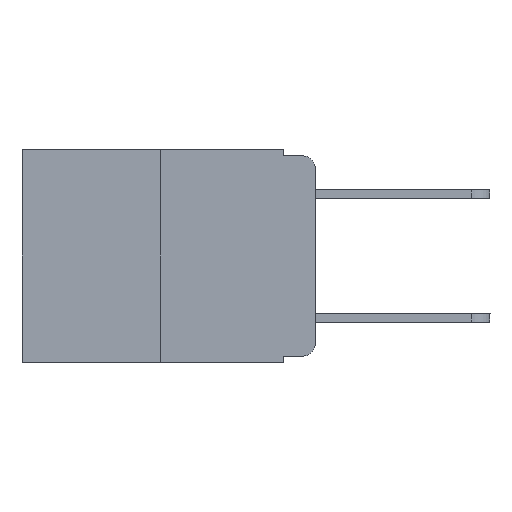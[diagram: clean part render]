
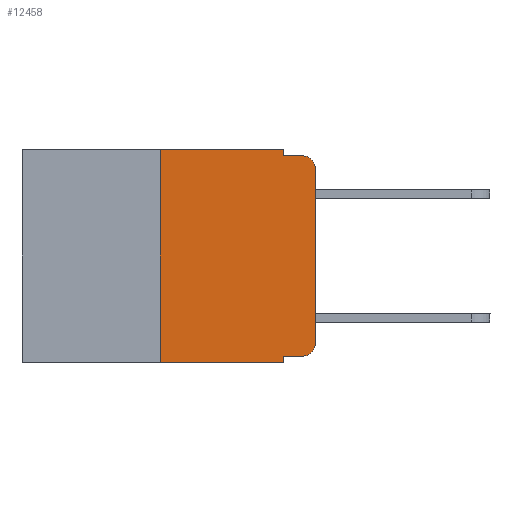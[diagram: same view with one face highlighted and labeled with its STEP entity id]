
A CAD part, left-side view. The second image highlights one B-rep face of the part: STEP entity #12458.
In plain terms, the highlighted planar face has unit normal (-1, 0, 0).
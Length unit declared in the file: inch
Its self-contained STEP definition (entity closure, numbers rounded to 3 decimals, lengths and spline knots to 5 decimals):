
#30 = ORIENTED_EDGE ( 'NONE', *, *, #13722, .T. ) ;
#354 = CARTESIAN_POINT ( 'NONE',  ( 0., 0.02, -0.03 ) ) ;
#429 = DIRECTION ( 'NONE',  ( 0., 0., -1. ) ) ;
#447 = CARTESIAN_POINT ( 'NONE',  ( 0., 0.473, -0.343 ) ) ;
#810 = EDGE_CURVE ( 'NONE', #1493, #2319, #4472, .T. ) ;
#872 = CARTESIAN_POINT ( 'NONE',  ( 0., 0.051, -0.333 ) ) ;
#1055 = VERTEX_POINT ( 'NONE', #14080 ) ;
#1112 = CARTESIAN_POINT ( 'NONE',  ( 0., 0.02, -0.313 ) ) ;
#1198 = DIRECTION ( 'NONE',  ( 1., 0., 0. ) ) ;
#1326 = VERTEX_POINT ( 'NONE', #9741 ) ;
#1418 = DIRECTION ( 'NONE',  ( 0., -1., 0. ) ) ;
#1493 = VERTEX_POINT ( 'NONE', #2427 ) ;
#2319 = VERTEX_POINT ( 'NONE', #12602 ) ;
#2427 = CARTESIAN_POINT ( 'NONE',  ( 0., 0.051, -0.01 ) ) ;
#2460 = LINE ( 'NONE', #447, #14008 ) ;
#2464 = CARTESIAN_POINT ( 'NONE',  ( 0., 0.02, -0.333 ) ) ;
#2469 = DIRECTION ( 'NONE',  ( 0., 0., -1. ) ) ;
#2837 = EDGE_CURVE ( 'NONE', #1326, #13571, #4199, .T. ) ;
#2861 = EDGE_CURVE ( 'NONE', #7603, #2319, #14036, .T. ) ;
#3283 = VERTEX_POINT ( 'NONE', #2464 ) ;
#3449 = ORIENTED_EDGE ( 'NONE', *, *, #3487, .T. ) ;
#3487 = EDGE_CURVE ( 'NONE', #16066, #7603, #9370, .T. ) ;
#3490 = VERTEX_POINT ( 'NONE', #7490 ) ;
#3627 = VECTOR ( 'NONE', #11086, 39.37008 ) ;
#3824 = CARTESIAN_POINT ( 'NONE',  ( 0., 0.051, 0. ) ) ;
#4148 = EDGE_LOOP ( 'NONE', ( #3449, #10349, #8048, #6821, #7260, #8786, #8287, #11688, #30, #13647 ) ) ;
#4199 = LINE ( 'NONE', #10698, #5879 ) ;
#4442 = DIRECTION ( 'NONE',  ( -1., 0., 0. ) ) ;
#4472 = LINE ( 'NONE', #9769, #3627 ) ;
#4588 = VECTOR ( 'NONE', #15865, 39.37008 ) ;
#4713 = DIRECTION ( 'NONE',  ( 0., 0., 1. ) ) ;
#4917 = EDGE_CURVE ( 'NONE', #3283, #16066, #12499, .T. ) ;
#5057 = LINE ( 'NONE', #7101, #6086 ) ;
#5068 = DIRECTION ( 'NONE',  ( 0., 0., -1. ) ) ;
#5173 = CARTESIAN_POINT ( 'NONE',  ( 0., 0., -0.313 ) ) ;
#5535 = FACE_OUTER_BOUND ( 'NONE', #4148, .T. ) ;
#5871 = AXIS2_PLACEMENT_3D ( 'NONE', #1112, #13280, #2469 ) ;
#5879 = VECTOR ( 'NONE', #1418, 39.37008 ) ;
#6086 = VECTOR ( 'NONE', #16521, 39.37008 ) ;
#6333 = LINE ( 'NONE', #13825, #13650 ) ;
#6821 = ORIENTED_EDGE ( 'NONE', *, *, #13826, .F. ) ;
#6951 = AXIS2_PLACEMENT_3D ( 'NONE', #354, #4442, #13757 ) ;
#7080 = DIRECTION ( 'NONE',  ( 0., -1., 0. ) ) ;
#7101 = CARTESIAN_POINT ( 'NONE',  ( 0., 0.25, 0. ) ) ;
#7260 = ORIENTED_EDGE ( 'NONE', *, *, #2837, .F. ) ;
#7490 = CARTESIAN_POINT ( 'NONE',  ( 0., 0.051, -0.343 ) ) ;
#7520 = AXIS2_PLACEMENT_3D ( 'NONE', #13140, #1198, #5068 ) ;
#7603 = VERTEX_POINT ( 'NONE', #12468 ) ;
#7617 = VERTEX_POINT ( 'NONE', #872 ) ;
#7890 = PLANE ( 'NONE',  #7520 ) ;
#8011 = DIRECTION ( 'NONE',  ( 0., -1., 0. ) ) ;
#8048 = ORIENTED_EDGE ( 'NONE', *, *, #810, .F. ) ;
#8287 = ORIENTED_EDGE ( 'NONE', *, *, #10129, .T. ) ;
#8550 = LINE ( 'NONE', #10136, #4588 ) ;
#8665 = CARTESIAN_POINT ( 'NONE',  ( 0., 0., 0. ) ) ;
#8786 = ORIENTED_EDGE ( 'NONE', *, *, #9233, .F. ) ;
#9233 = EDGE_CURVE ( 'NONE', #1055, #1326, #5057, .T. ) ;
#9370 = LINE ( 'NONE', #8665, #11711 ) ;
#9579 = EDGE_CURVE ( 'NONE', #7617, #3490, #8550, .T. ) ;
#9741 = CARTESIAN_POINT ( 'NONE',  ( 0., 0.25, 0. ) ) ;
#9769 = CARTESIAN_POINT ( 'NONE',  ( 0., 0.051, -0.01 ) ) ;
#10129 = EDGE_CURVE ( 'NONE', #1055, #3490, #2460, .T. ) ;
#10136 = CARTESIAN_POINT ( 'NONE',  ( 0., 0.051, 0. ) ) ;
#10349 = ORIENTED_EDGE ( 'NONE', *, *, #2861, .T. ) ;
#10698 = CARTESIAN_POINT ( 'NONE',  ( 0., 0.473, 0. ) ) ;
#11086 = DIRECTION ( 'NONE',  ( 0., -1., 0. ) ) ;
#11688 = ORIENTED_EDGE ( 'NONE', *, *, #9579, .F. ) ;
#11711 = VECTOR ( 'NONE', #4713, 39.37008 ) ;
#12458 = ADVANCED_FACE ( 'NONE', ( #5535 ), #7890, .F. ) ;
#12468 = CARTESIAN_POINT ( 'NONE',  ( 0., 0., -0.03 ) ) ;
#12499 = CIRCLE ( 'NONE', #5871, 0.02 ) ;
#12602 = CARTESIAN_POINT ( 'NONE',  ( 0., 0.02, -0.01 ) ) ;
#12811 = VECTOR ( 'NONE', #8011, 39.37008 ) ;
#13140 = CARTESIAN_POINT ( 'NONE',  ( 0., 0.473, 0. ) ) ;
#13280 = DIRECTION ( 'NONE',  ( -1., 0., 0. ) ) ;
#13571 = VERTEX_POINT ( 'NONE', #3824 ) ;
#13594 = CARTESIAN_POINT ( 'NONE',  ( 0., 0.051, -0.333 ) ) ;
#13647 = ORIENTED_EDGE ( 'NONE', *, *, #4917, .T. ) ;
#13650 = VECTOR ( 'NONE', #429, 39.37008 ) ;
#13722 = EDGE_CURVE ( 'NONE', #7617, #3283, #14904, .T. ) ;
#13757 = DIRECTION ( 'NONE',  ( 0., 0., -1. ) ) ;
#13825 = CARTESIAN_POINT ( 'NONE',  ( 0., 0.051, 0. ) ) ;
#13826 = EDGE_CURVE ( 'NONE', #13571, #1493, #6333, .T. ) ;
#14008 = VECTOR ( 'NONE', #7080, 39.37008 ) ;
#14036 = CIRCLE ( 'NONE', #6951, 0.02 ) ;
#14080 = CARTESIAN_POINT ( 'NONE',  ( 0., 0.25, -0.343 ) ) ;
#14904 = LINE ( 'NONE', #13594, #12811 ) ;
#15865 = DIRECTION ( 'NONE',  ( 0., 0., -1. ) ) ;
#16066 = VERTEX_POINT ( 'NONE', #5173 ) ;
#16521 = DIRECTION ( 'NONE',  ( 0., 0., 1. ) ) ;
